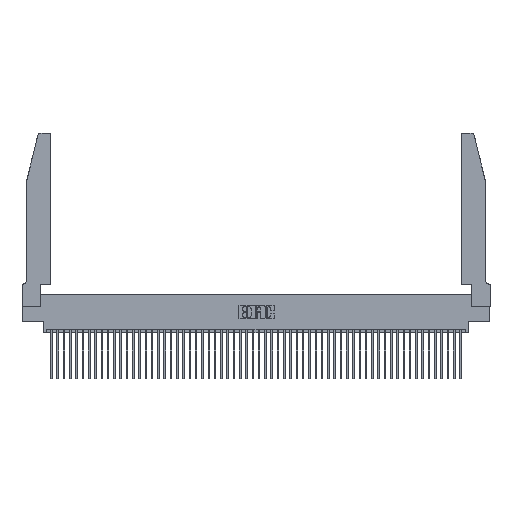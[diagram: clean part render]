
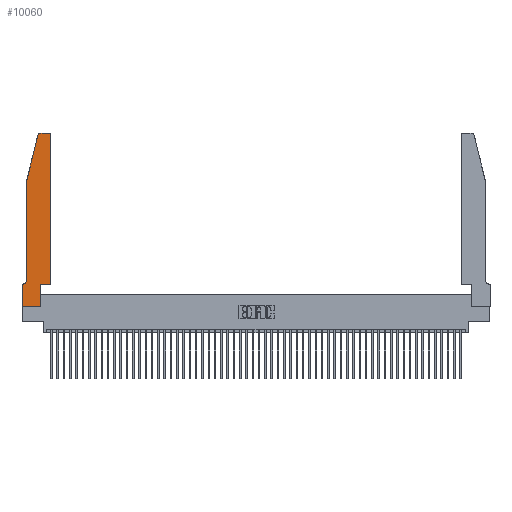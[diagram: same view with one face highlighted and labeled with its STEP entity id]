
A CAD part, top view. The second image highlights one B-rep face of the part: STEP entity #10060.
In plain terms, the highlighted planar face has unit normal (0, 0, 1).
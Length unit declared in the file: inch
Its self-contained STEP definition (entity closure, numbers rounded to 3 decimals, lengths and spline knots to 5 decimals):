
#504 = ORIENTED_EDGE ( 'NONE', *, *, #38425, .T. ) ;
#610 = EDGE_CURVE ( 'NONE', #37981, #47244, #9296, .T. ) ;
#755 = CIRCLE ( 'NONE', #26322, 0.03 ) ;
#1986 = CARTESIAN_POINT ( 'NONE',  ( 0.4205, 2.75, 0.37 ) ) ;
#3117 = AXIS2_PLACEMENT_3D ( 'NONE', #4632, #8825, #37774 ) ;
#3710 = CARTESIAN_POINT ( 'NONE',  ( 0.284, 2.75, 0.37 ) ) ;
#4082 = EDGE_CURVE ( 'NONE', #45464, #4616, #38508, .T. ) ;
#4616 = VERTEX_POINT ( 'NONE', #24112 ) ;
#4632 = CARTESIAN_POINT ( 'NONE',  ( 0., 0.35, 0.37 ) ) ;
#4787 = VECTOR ( 'NONE', #22024, 39.37008 ) ;
#4870 = EDGE_CURVE ( 'NONE', #47244, #11003, #755, .T. ) ;
#5089 = DIRECTION ( 'NONE',  ( 0., 0., 1. ) ) ;
#5392 = EDGE_LOOP ( 'NONE', ( #21779, #46019, #32831, #37314, #13124, #33606, #28834, #30757, #10733, #504, #10253, #42261 ) ) ;
#6738 = CARTESIAN_POINT ( 'NONE',  ( 0.2865, 0.35, 0.37 ) ) ;
#6805 = VECTOR ( 'NONE', #7764, 39.37008 ) ;
#6952 = VECTOR ( 'NONE', #27645, 39.37008 ) ;
#6985 = CIRCLE ( 'NONE', #28579, 0.03 ) ;
#7764 = DIRECTION ( 'NONE',  ( 1., 0., 0. ) ) ;
#8825 = DIRECTION ( 'NONE',  ( 0., 0., 1. ) ) ;
#9203 = EDGE_CURVE ( 'NONE', #38713, #42798, #6985, .T. ) ;
#9296 = LINE ( 'NONE', #29600, #17802 ) ;
#9401 = EDGE_CURVE ( 'NONE', #33455, #23335, #50147, .T. ) ;
#9758 = DIRECTION ( 'NONE',  ( 0., 0., 1. ) ) ;
#10060 = ADVANCED_FACE ( 'NONE', ( #20600 ), #41721, .T. ) ;
#10253 = ORIENTED_EDGE ( 'NONE', *, *, #610, .T. ) ;
#10733 = ORIENTED_EDGE ( 'NONE', *, *, #21851, .T. ) ;
#11003 = VERTEX_POINT ( 'NONE', #1986 ) ;
#11910 = CIRCLE ( 'NONE', #15250, 0.07 ) ;
#13124 = ORIENTED_EDGE ( 'NONE', *, *, #39453, .T. ) ;
#14862 = CARTESIAN_POINT ( 'NONE',  ( 0.0755, 2., 0.37 ) ) ;
#15250 = AXIS2_PLACEMENT_3D ( 'NONE', #16597, #45392, #20811 ) ;
#16097 = VECTOR ( 'NONE', #39916, 39.37008 ) ;
#16597 = CARTESIAN_POINT ( 'NONE',  ( 0.0055, 0.42, 0.37 ) ) ;
#16978 = CARTESIAN_POINT ( 'NONE',  ( 0., 0.35, 0.37 ) ) ;
#17802 = VECTOR ( 'NONE', #49950, 39.37008 ) ;
#18061 = VECTOR ( 'NONE', #43697, 39.37008 ) ;
#20286 = CARTESIAN_POINT ( 'NONE',  ( 0., 0., 0.37 ) ) ;
#20600 = FACE_OUTER_BOUND ( 'NONE', #5392, .T. ) ;
#20698 = VECTOR ( 'NONE', #32013, 39.37008 ) ;
#20811 = DIRECTION ( 'NONE',  ( -1., 0., 0. ) ) ;
#21443 = VERTEX_POINT ( 'NONE', #16978 ) ;
#21779 = ORIENTED_EDGE ( 'NONE', *, *, #22264, .T. ) ;
#21851 = EDGE_CURVE ( 'NONE', #4616, #23540, #52059, .T. ) ;
#22024 = DIRECTION ( 'NONE',  ( 1., 0., 0. ) ) ;
#22264 = EDGE_CURVE ( 'NONE', #11003, #38713, #25190, .T. ) ;
#23335 = VERTEX_POINT ( 'NONE', #37782 ) ;
#23540 = VERTEX_POINT ( 'NONE', #39549 ) ;
#23675 = EDGE_CURVE ( 'NONE', #25519, #21443, #31642, .T. ) ;
#24112 = CARTESIAN_POINT ( 'NONE',  ( 0.2865, 0., 0.37 ) ) ;
#24527 = VECTOR ( 'NONE', #33598, 39.37008 ) ;
#25190 = LINE ( 'NONE', #46636, #45690 ) ;
#25519 = VERTEX_POINT ( 'NONE', #30611 ) ;
#26322 = AXIS2_PLACEMENT_3D ( 'NONE', #29994, #5089, #34097 ) ;
#27645 = DIRECTION ( 'NONE',  ( 0., 1., 0. ) ) ;
#28579 = AXIS2_PLACEMENT_3D ( 'NONE', #34562, #9758, #38664 ) ;
#28834 = ORIENTED_EDGE ( 'NONE', *, *, #37100, .T. ) ;
#29507 = CARTESIAN_POINT ( 'NONE',  ( 0., 0., 0.37 ) ) ;
#29600 = CARTESIAN_POINT ( 'NONE',  ( 0.4505, 0.35, 0.37 ) ) ;
#29994 = CARTESIAN_POINT ( 'NONE',  ( 0.4205, 2.72, 0.37 ) ) ;
#30422 = CARTESIAN_POINT ( 'NONE',  ( 0.0755, 2., 0.37 ) ) ;
#30611 = CARTESIAN_POINT ( 'NONE',  ( 0.0055, 0.35, 0.37 ) ) ;
#30757 = ORIENTED_EDGE ( 'NONE', *, *, #4082, .T. ) ;
#31642 = LINE ( 'NONE', #44238, #20698 ) ;
#32013 = DIRECTION ( 'NONE',  ( -1., 0., 0. ) ) ;
#32831 = ORIENTED_EDGE ( 'NONE', *, *, #45259, .T. ) ;
#33455 = VERTEX_POINT ( 'NONE', #30422 ) ;
#33598 = DIRECTION ( 'NONE',  ( 0., -1., 0. ) ) ;
#33606 = ORIENTED_EDGE ( 'NONE', *, *, #23675, .T. ) ;
#34097 = DIRECTION ( 'NONE',  ( 1., 0., 0. ) ) ;
#34562 = CARTESIAN_POINT ( 'NONE',  ( 0.284, 2.72, 0.37 ) ) ;
#35434 = LINE ( 'NONE', #29507, #24527 ) ;
#35696 = CARTESIAN_POINT ( 'NONE',  ( 0.4505, 0.35, 0.37 ) ) ;
#37100 = EDGE_CURVE ( 'NONE', #21443, #45464, #35434, .T. ) ;
#37314 = ORIENTED_EDGE ( 'NONE', *, *, #9401, .T. ) ;
#37774 = DIRECTION ( 'NONE',  ( 1., 0., 0. ) ) ;
#37782 = CARTESIAN_POINT ( 'NONE',  ( 0.0755, 0.42, 0.37 ) ) ;
#37981 = VERTEX_POINT ( 'NONE', #35696 ) ;
#38045 = CARTESIAN_POINT ( 'NONE',  ( 0.4505, 2.72, 0.37 ) ) ;
#38425 = EDGE_CURVE ( 'NONE', #23540, #37981, #48714, .T. ) ;
#38508 = LINE ( 'NONE', #49018, #6805 ) ;
#38664 = DIRECTION ( 'NONE',  ( 1., 0., 0. ) ) ;
#38713 = VERTEX_POINT ( 'NONE', #3710 ) ;
#39453 = EDGE_CURVE ( 'NONE', #23335, #25519, #11910, .T. ) ;
#39549 = CARTESIAN_POINT ( 'NONE',  ( 0.2865, 0.35, 0.37 ) ) ;
#39916 = DIRECTION ( 'NONE',  ( 0., -1., 0. ) ) ;
#40682 = CARTESIAN_POINT ( 'NONE',  ( 0.25487, 2.72718, 0.37 ) ) ;
#41721 = PLANE ( 'NONE',  #3117 ) ;
#42261 = ORIENTED_EDGE ( 'NONE', *, *, #4870, .T. ) ;
#42798 = VERTEX_POINT ( 'NONE', #40682 ) ;
#43697 = DIRECTION ( 'NONE',  ( -0.239, -0.971, 0. ) ) ;
#44238 = CARTESIAN_POINT ( 'NONE',  ( 0.0755, 0.35, 0.37 ) ) ;
#45259 = EDGE_CURVE ( 'NONE', #42798, #33455, #49513, .T. ) ;
#45392 = DIRECTION ( 'NONE',  ( 0., 0., -1. ) ) ;
#45464 = VERTEX_POINT ( 'NONE', #20286 ) ;
#45690 = VECTOR ( 'NONE', #50731, 39.37008 ) ;
#46019 = ORIENTED_EDGE ( 'NONE', *, *, #9203, .T. ) ;
#46636 = CARTESIAN_POINT ( 'NONE',  ( 0.2605, 2.75, 0.37 ) ) ;
#47244 = VERTEX_POINT ( 'NONE', #38045 ) ;
#48714 = LINE ( 'NONE', #50469, #4787 ) ;
#49018 = CARTESIAN_POINT ( 'NONE',  ( 0., 0., 0.37 ) ) ;
#49513 = LINE ( 'NONE', #14862, #18061 ) ;
#49950 = DIRECTION ( 'NONE',  ( 0., 1., 0. ) ) ;
#50147 = LINE ( 'NONE', #52027, #16097 ) ;
#50469 = CARTESIAN_POINT ( 'NONE',  ( 0.4505, 0.35, 0.37 ) ) ;
#50731 = DIRECTION ( 'NONE',  ( -1., 0., 0. ) ) ;
#52027 = CARTESIAN_POINT ( 'NONE',  ( 0.0755, 2., 0.37 ) ) ;
#52059 = LINE ( 'NONE', #6738, #6952 ) ;
